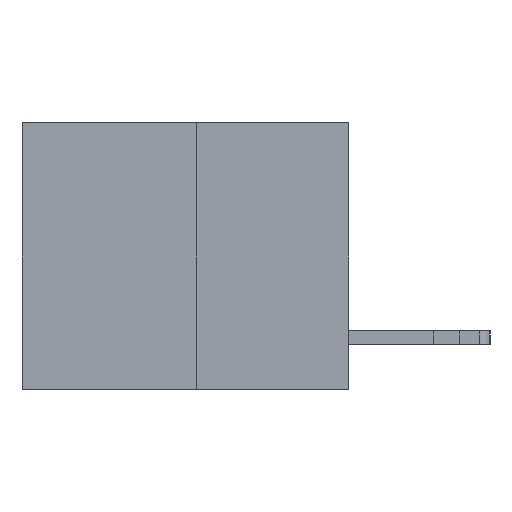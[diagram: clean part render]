
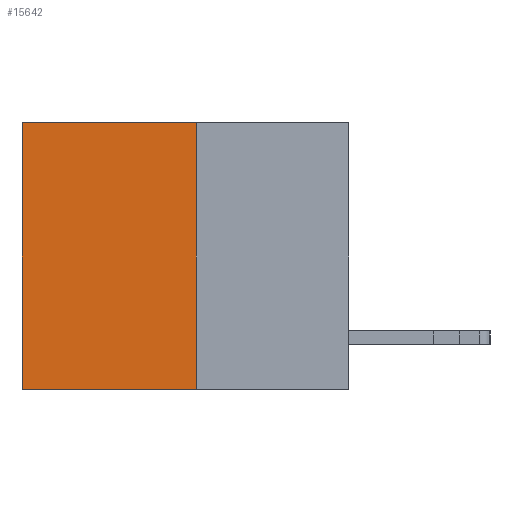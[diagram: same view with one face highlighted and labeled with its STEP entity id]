
A CAD part, left-side view. The second image highlights one B-rep face of the part: STEP entity #15642.
In plain terms, the highlighted planar face has unit normal (-1, 0, 0).
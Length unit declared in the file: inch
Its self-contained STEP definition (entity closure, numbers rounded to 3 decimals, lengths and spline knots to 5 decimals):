
#146 = VERTEX_POINT ( 'NONE', #12679 ) ;
#232 = EDGE_CURVE ( 'NONE', #146, #10085, #3095, .T. ) ;
#784 = DIRECTION ( 'NONE',  ( 0., 1., 0. ) ) ;
#1467 = CARTESIAN_POINT ( 'NONE',  ( 0.3165, 0.28, -0.49 ) ) ;
#2154 = FACE_OUTER_BOUND ( 'NONE', #14004, .T. ) ;
#2569 = LINE ( 'NONE', #5955, #4490 ) ;
#2652 = CARTESIAN_POINT ( 'NONE',  ( 0.3165, 0.6, 0. ) ) ;
#2742 = CARTESIAN_POINT ( 'NONE',  ( 0.3165, 0.28, -0.49 ) ) ;
#3095 = LINE ( 'NONE', #2742, #12559 ) ;
#3222 = DIRECTION ( 'NONE',  ( 0., 0., -1. ) ) ;
#3390 = LINE ( 'NONE', #4401, #15781 ) ;
#3623 = PLANE ( 'NONE',  #4773 ) ;
#4401 = CARTESIAN_POINT ( 'NONE',  ( 0.3165, 0.28, -0.49 ) ) ;
#4490 = VECTOR ( 'NONE', #14618, 39.37008 ) ;
#4773 = AXIS2_PLACEMENT_3D ( 'NONE', #14770, #4922, #7413 ) ;
#4922 = DIRECTION ( 'NONE',  ( 1., 0., 0. ) ) ;
#5041 = ORIENTED_EDGE ( 'NONE', *, *, #5638, .T. ) ;
#5638 = EDGE_CURVE ( 'NONE', #7361, #6812, #13221, .T. ) ;
#5676 = VECTOR ( 'NONE', #3222, 39.37008 ) ;
#5955 = CARTESIAN_POINT ( 'NONE',  ( 0.3165, 0.28, 0. ) ) ;
#5995 = CARTESIAN_POINT ( 'NONE',  ( 0.3165, 0.6, -0.49 ) ) ;
#6812 = VERTEX_POINT ( 'NONE', #5995 ) ;
#7075 = ORIENTED_EDGE ( 'NONE', *, *, #232, .F. ) ;
#7361 = VERTEX_POINT ( 'NONE', #2652 ) ;
#7382 = ORIENTED_EDGE ( 'NONE', *, *, #11901, .T. ) ;
#7413 = DIRECTION ( 'NONE',  ( 0., 0., -1. ) ) ;
#8880 = DIRECTION ( 'NONE',  ( 0., 0., -1. ) ) ;
#9400 = CARTESIAN_POINT ( 'NONE',  ( 0.3165, 0.6, -0.49 ) ) ;
#9834 = EDGE_CURVE ( 'NONE', #10085, #6812, #3390, .T. ) ;
#10085 = VERTEX_POINT ( 'NONE', #1467 ) ;
#11901 = EDGE_CURVE ( 'NONE', #146, #7361, #2569, .T. ) ;
#12261 = ORIENTED_EDGE ( 'NONE', *, *, #9834, .F. ) ;
#12559 = VECTOR ( 'NONE', #8880, 39.37008 ) ;
#12679 = CARTESIAN_POINT ( 'NONE',  ( 0.3165, 0.28, 0. ) ) ;
#13221 = LINE ( 'NONE', #9400, #5676 ) ;
#14004 = EDGE_LOOP ( 'NONE', ( #5041, #12261, #7075, #7382 ) ) ;
#14618 = DIRECTION ( 'NONE',  ( 0., 1., 0. ) ) ;
#14770 = CARTESIAN_POINT ( 'NONE',  ( 0.3165, 0.28, -0.49 ) ) ;
#15642 = ADVANCED_FACE ( 'NONE', ( #2154 ), #3623, .F. ) ;
#15781 = VECTOR ( 'NONE', #784, 39.37008 ) ;
